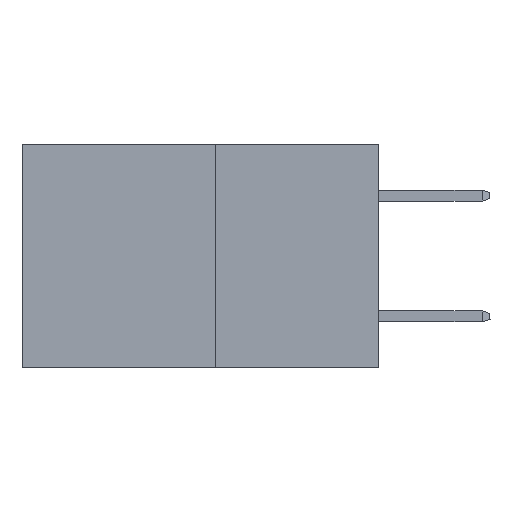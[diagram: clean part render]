
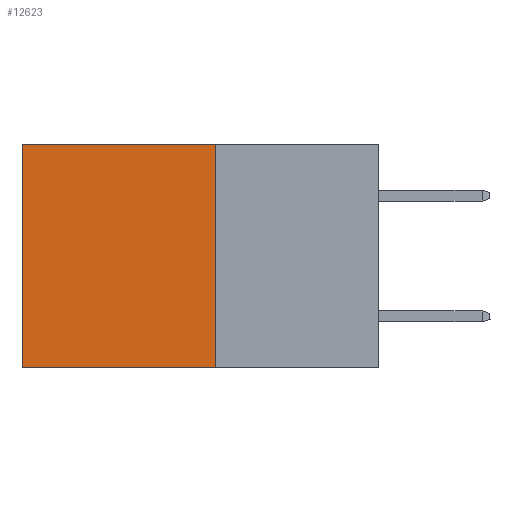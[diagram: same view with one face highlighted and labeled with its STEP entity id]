
A CAD part, left-side view. The second image highlights one B-rep face of the part: STEP entity #12623.
In plain terms, the highlighted planar face has unit normal (-1, 0, 0).
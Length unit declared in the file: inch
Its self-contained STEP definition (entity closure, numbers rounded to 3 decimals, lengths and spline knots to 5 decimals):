
#173 = CARTESIAN_POINT ( 'NONE',  ( 0.277, 0.59, -0.37 ) ) ;
#534 = ORIENTED_EDGE ( 'NONE', *, *, #8578, .F. ) ;
#659 = ORIENTED_EDGE ( 'NONE', *, *, #1921, .F. ) ;
#728 = ORIENTED_EDGE ( 'NONE', *, *, #18525, .T. ) ;
#758 = ORIENTED_EDGE ( 'NONE', *, *, #9844, .T. ) ;
#1793 = LINE ( 'NONE', #8329, #9507 ) ;
#1921 = EDGE_CURVE ( 'NONE', #6476, #16451, #1793, .T. ) ;
#2169 = VECTOR ( 'NONE', #7343, 39.37008 ) ;
#3251 = DIRECTION ( 'NONE',  ( 0., 1., 0. ) ) ;
#4037 = CARTESIAN_POINT ( 'NONE',  ( 0.277, 0.27, -0.37 ) ) ;
#4094 = FACE_OUTER_BOUND ( 'NONE', #7891, .T. ) ;
#4297 = VERTEX_POINT ( 'NONE', #18399 ) ;
#6476 = VERTEX_POINT ( 'NONE', #14493 ) ;
#7343 = DIRECTION ( 'NONE',  ( 0., 0., -1. ) ) ;
#7891 = EDGE_LOOP ( 'NONE', ( #728, #534, #659, #758 ) ) ;
#8329 = CARTESIAN_POINT ( 'NONE',  ( 0.277, 0.27, -0.37 ) ) ;
#8477 = DIRECTION ( 'NONE',  ( 0., 1., 0. ) ) ;
#8538 = CARTESIAN_POINT ( 'NONE',  ( 0.277, 0.27, 0. ) ) ;
#8578 = EDGE_CURVE ( 'NONE', #16451, #13467, #9349, .T. ) ;
#9042 = DIRECTION ( 'NONE',  ( 1., 0., 0. ) ) ;
#9349 = LINE ( 'NONE', #4037, #16627 ) ;
#9507 = VECTOR ( 'NONE', #11582, 39.37008 ) ;
#9730 = LINE ( 'NONE', #8538, #13700 ) ;
#9844 = EDGE_CURVE ( 'NONE', #6476, #4297, #9730, .T. ) ;
#10364 = LINE ( 'NONE', #17513, #2169 ) ;
#11582 = DIRECTION ( 'NONE',  ( 0., 0., -1. ) ) ;
#11951 = PLANE ( 'NONE',  #13539 ) ;
#12623 = ADVANCED_FACE ( 'NONE', ( #4094 ), #11951, .F. ) ;
#13467 = VERTEX_POINT ( 'NONE', #173 ) ;
#13539 = AXIS2_PLACEMENT_3D ( 'NONE', #17713, #9042, #19164 ) ;
#13700 = VECTOR ( 'NONE', #8477, 39.37008 ) ;
#14185 = CARTESIAN_POINT ( 'NONE',  ( 0.277, 0.27, -0.37 ) ) ;
#14493 = CARTESIAN_POINT ( 'NONE',  ( 0.277, 0.27, 0. ) ) ;
#16451 = VERTEX_POINT ( 'NONE', #14185 ) ;
#16627 = VECTOR ( 'NONE', #3251, 39.37008 ) ;
#17513 = CARTESIAN_POINT ( 'NONE',  ( 0.277, 0.59, -0.37 ) ) ;
#17713 = CARTESIAN_POINT ( 'NONE',  ( 0.277, 0.27, -0.37 ) ) ;
#18399 = CARTESIAN_POINT ( 'NONE',  ( 0.277, 0.59, 0. ) ) ;
#18525 = EDGE_CURVE ( 'NONE', #4297, #13467, #10364, .T. ) ;
#19164 = DIRECTION ( 'NONE',  ( 0., 0., -1. ) ) ;
